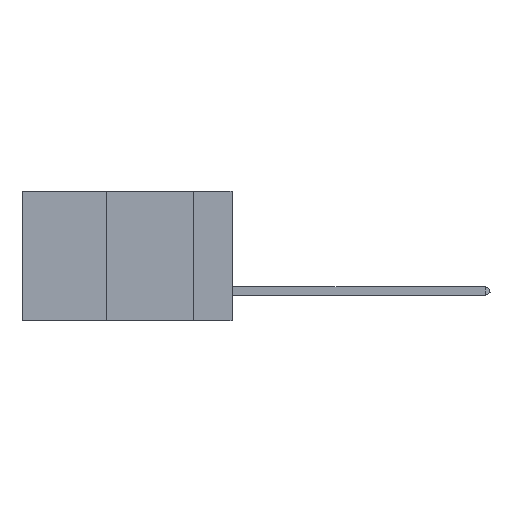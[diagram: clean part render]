
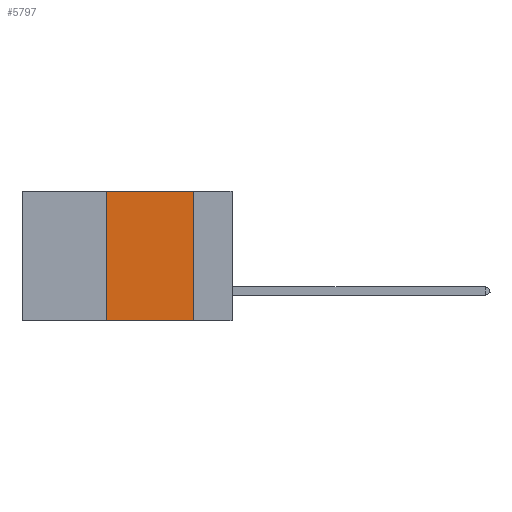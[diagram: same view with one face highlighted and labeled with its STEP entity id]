
A CAD part, left-side view. The second image highlights one B-rep face of the part: STEP entity #5797.
In plain terms, the highlighted planar face has unit normal (-1, 0, 0).
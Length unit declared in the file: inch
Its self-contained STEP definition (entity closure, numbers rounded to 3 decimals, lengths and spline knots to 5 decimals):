
#653 = EDGE_CURVE ( 'NONE', #17035, #6031, #17224, .T. ) ;
#801 = DIRECTION ( 'NONE',  ( 0., -1., 0. ) ) ;
#1124 = CARTESIAN_POINT ( 'NONE',  ( 0., 0.36, -0.37 ) ) ;
#1419 = EDGE_CURVE ( 'NONE', #16702, #3063, #9067, .T. ) ;
#1791 = DIRECTION ( 'NONE',  ( 0., 0., 1. ) ) ;
#1962 = LINE ( 'NONE', #14263, #12806 ) ;
#2434 = EDGE_CURVE ( 'NONE', #6031, #16702, #1962, .T. ) ;
#2634 = CARTESIAN_POINT ( 'NONE',  ( 0., 0.11, 0. ) ) ;
#2690 = DIRECTION ( 'NONE',  ( 0., -1., 0. ) ) ;
#3063 = VERTEX_POINT ( 'NONE', #15061 ) ;
#3731 = PLANE ( 'NONE',  #17295 ) ;
#4712 = DIRECTION ( 'NONE',  ( 0., 0., -1. ) ) ;
#5071 = CARTESIAN_POINT ( 'NONE',  ( 0., 0.6, 0. ) ) ;
#5313 = CARTESIAN_POINT ( 'NONE',  ( 0., 0.6, -0.37 ) ) ;
#5797 = ADVANCED_FACE ( 'NONE', ( #8739 ), #3731, .F. ) ;
#6031 = VERTEX_POINT ( 'NONE', #15530 ) ;
#6299 = VECTOR ( 'NONE', #2690, 39.37008 ) ;
#6523 = ORIENTED_EDGE ( 'NONE', *, *, #2434, .F. ) ;
#7345 = CARTESIAN_POINT ( 'NONE',  ( 0., 0.36, 0. ) ) ;
#8455 = VECTOR ( 'NONE', #1791, 39.37008 ) ;
#8644 = VECTOR ( 'NONE', #4712, 39.37008 ) ;
#8739 = FACE_OUTER_BOUND ( 'NONE', #11861, .T. ) ;
#9067 = LINE ( 'NONE', #9851, #8644 ) ;
#9179 = ORIENTED_EDGE ( 'NONE', *, *, #1419, .F. ) ;
#9212 = DIRECTION ( 'NONE',  ( 1., 0., 0. ) ) ;
#9851 = CARTESIAN_POINT ( 'NONE',  ( 0., 0.11, 0. ) ) ;
#10816 = ORIENTED_EDGE ( 'NONE', *, *, #16749, .T. ) ;
#11861 = EDGE_LOOP ( 'NONE', ( #9179, #6523, #16054, #10816 ) ) ;
#12083 = DIRECTION ( 'NONE',  ( 0., 0., -1. ) ) ;
#12806 = VECTOR ( 'NONE', #801, 39.37008 ) ;
#14263 = CARTESIAN_POINT ( 'NONE',  ( 0., 0.6, 0. ) ) ;
#14443 = LINE ( 'NONE', #5313, #6299 ) ;
#15061 = CARTESIAN_POINT ( 'NONE',  ( 0., 0.11, -0.37 ) ) ;
#15530 = CARTESIAN_POINT ( 'NONE',  ( 0., 0.36, 0. ) ) ;
#16054 = ORIENTED_EDGE ( 'NONE', *, *, #653, .F. ) ;
#16702 = VERTEX_POINT ( 'NONE', #2634 ) ;
#16749 = EDGE_CURVE ( 'NONE', #17035, #3063, #14443, .T. ) ;
#17035 = VERTEX_POINT ( 'NONE', #1124 ) ;
#17224 = LINE ( 'NONE', #7345, #8455 ) ;
#17295 = AXIS2_PLACEMENT_3D ( 'NONE', #5071, #9212, #12083 ) ;
